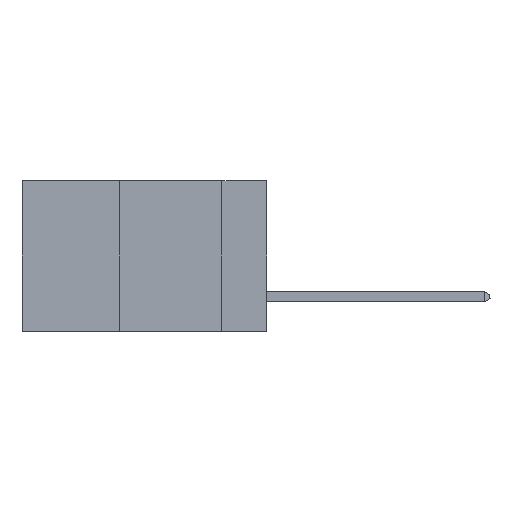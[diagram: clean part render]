
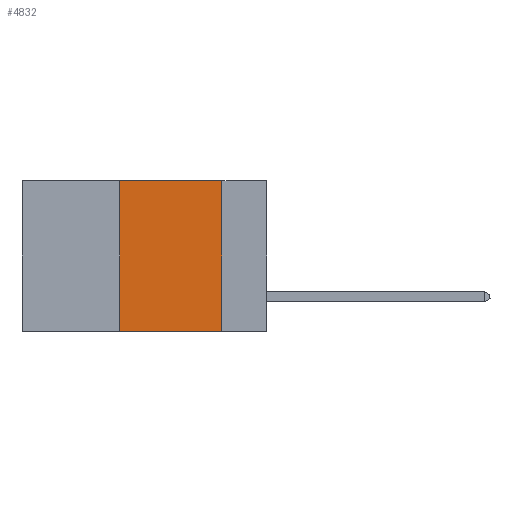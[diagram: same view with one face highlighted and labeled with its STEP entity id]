
A CAD part, left-side view. The second image highlights one B-rep face of the part: STEP entity #4832.
In plain terms, the highlighted planar face has unit normal (-1, 0, 0).
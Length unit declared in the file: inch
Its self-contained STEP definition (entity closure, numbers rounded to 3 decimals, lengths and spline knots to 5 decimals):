
#249 = VERTEX_POINT ( 'NONE', #8306 ) ;
#294 = AXIS2_PLACEMENT_3D ( 'NONE', #7048, #3923, #2354 ) ;
#620 = FACE_OUTER_BOUND ( 'NONE', #8728, .T. ) ;
#1082 = EDGE_CURVE ( 'NONE', #249, #7417, #6162, .T. ) ;
#1263 = VECTOR ( 'NONE', #8665, 39.37008 ) ;
#1742 = LINE ( 'NONE', #10093, #9099 ) ;
#1938 = VERTEX_POINT ( 'NONE', #5093 ) ;
#2170 = CARTESIAN_POINT ( 'NONE',  ( 0., 0.6, 0. ) ) ;
#2354 = DIRECTION ( 'NONE',  ( 0., 0., -1. ) ) ;
#3054 = CARTESIAN_POINT ( 'NONE',  ( 0., 0.11, -0.37 ) ) ;
#3196 = CARTESIAN_POINT ( 'NONE',  ( 0., 0.36, 0. ) ) ;
#3354 = DIRECTION ( 'NONE',  ( 0., 0., -1. ) ) ;
#3359 = VECTOR ( 'NONE', #3354, 39.37008 ) ;
#3614 = EDGE_CURVE ( 'NONE', #249, #7330, #1742, .T. ) ;
#3727 = DIRECTION ( 'NONE',  ( 0., -1., 0. ) ) ;
#3829 = DIRECTION ( 'NONE',  ( 0., -1., 0. ) ) ;
#3845 = LINE ( 'NONE', #4101, #3359 ) ;
#3923 = DIRECTION ( 'NONE',  ( 1., 0., 0. ) ) ;
#4101 = CARTESIAN_POINT ( 'NONE',  ( 0., 0.11, 0. ) ) ;
#4138 = VECTOR ( 'NONE', #3727, 39.37008 ) ;
#4546 = EDGE_CURVE ( 'NONE', #7417, #1938, #7822, .T. ) ;
#4832 = ADVANCED_FACE ( 'NONE', ( #620 ), #9278, .F. ) ;
#5093 = CARTESIAN_POINT ( 'NONE',  ( 0., 0.11, 0. ) ) ;
#5523 = ORIENTED_EDGE ( 'NONE', *, *, #7906, .F. ) ;
#6162 = LINE ( 'NONE', #8568, #1263 ) ;
#7048 = CARTESIAN_POINT ( 'NONE',  ( 0., 0.6, 0. ) ) ;
#7330 = VERTEX_POINT ( 'NONE', #3054 ) ;
#7397 = ORIENTED_EDGE ( 'NONE', *, *, #1082, .F. ) ;
#7417 = VERTEX_POINT ( 'NONE', #3196 ) ;
#7822 = LINE ( 'NONE', #2170, #4138 ) ;
#7906 = EDGE_CURVE ( 'NONE', #1938, #7330, #3845, .T. ) ;
#8306 = CARTESIAN_POINT ( 'NONE',  ( 0., 0.36, -0.37 ) ) ;
#8437 = ORIENTED_EDGE ( 'NONE', *, *, #3614, .T. ) ;
#8568 = CARTESIAN_POINT ( 'NONE',  ( 0., 0.36, 0. ) ) ;
#8665 = DIRECTION ( 'NONE',  ( 0., 0., 1. ) ) ;
#8728 = EDGE_LOOP ( 'NONE', ( #5523, #9061, #7397, #8437 ) ) ;
#9061 = ORIENTED_EDGE ( 'NONE', *, *, #4546, .F. ) ;
#9099 = VECTOR ( 'NONE', #3829, 39.37008 ) ;
#9278 = PLANE ( 'NONE',  #294 ) ;
#10093 = CARTESIAN_POINT ( 'NONE',  ( 0., 0.6, -0.37 ) ) ;
